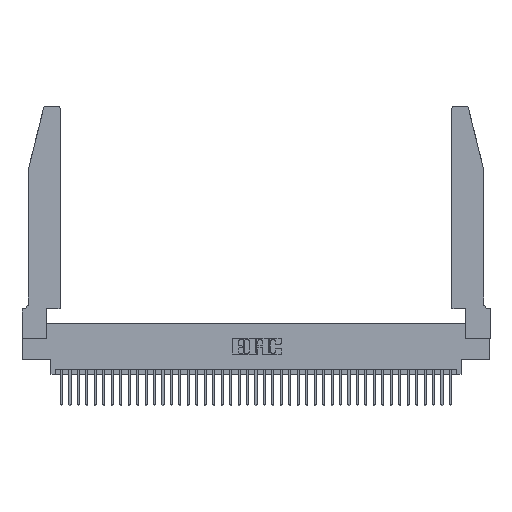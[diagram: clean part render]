
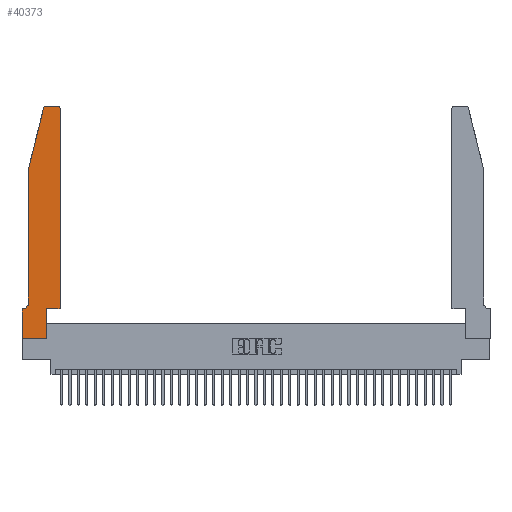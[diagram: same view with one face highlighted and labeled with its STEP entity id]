
A CAD part, top view. The second image highlights one B-rep face of the part: STEP entity #40373.
In plain terms, the highlighted planar face has unit normal (0, 0, 1).
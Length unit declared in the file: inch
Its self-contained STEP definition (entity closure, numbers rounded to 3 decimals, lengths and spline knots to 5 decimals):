
#163 = EDGE_CURVE ( 'NONE', #26604, #31561, #27139, .T. ) ;
#851 = DIRECTION ( 'NONE',  ( 0., -1., 0. ) ) ;
#1179 = AXIS2_PLACEMENT_3D ( 'NONE', #20336, #20608, #15203 ) ;
#2220 = CARTESIAN_POINT ( 'NONE',  ( 0.4505, 0.35, 0.37 ) ) ;
#2882 = VECTOR ( 'NONE', #851, 39.37008 ) ;
#3058 = ORIENTED_EDGE ( 'NONE', *, *, #35849, .T. ) ;
#3100 = ORIENTED_EDGE ( 'NONE', *, *, #12006, .T. ) ;
#3181 = VECTOR ( 'NONE', #8844, 39.37008 ) ;
#3531 = AXIS2_PLACEMENT_3D ( 'NONE', #12053, #40711, #15668 ) ;
#4727 = CIRCLE ( 'NONE', #17634, 0.03 ) ;
#4817 = LINE ( 'NONE', #2220, #30569 ) ;
#6264 = EDGE_CURVE ( 'NONE', #33062, #15789, #32249, .T. ) ;
#8247 = FACE_OUTER_BOUND ( 'NONE', #38529, .T. ) ;
#8464 = CARTESIAN_POINT ( 'NONE',  ( 0.2865, 0.35, 0.37 ) ) ;
#8844 = DIRECTION ( 'NONE',  ( -0.239, -0.971, 0. ) ) ;
#9478 = DIRECTION ( 'NONE',  ( 0., 0., 1. ) ) ;
#9781 = LINE ( 'NONE', #20766, #28170 ) ;
#10214 = CARTESIAN_POINT ( 'NONE',  ( 0.2865, 0., 0.37 ) ) ;
#10306 = ORIENTED_EDGE ( 'NONE', *, *, #33803, .T. ) ;
#11037 = EDGE_CURVE ( 'NONE', #12866, #26750, #38738, .T. ) ;
#11564 = LINE ( 'NONE', #15688, #3181 ) ;
#11738 = CARTESIAN_POINT ( 'NONE',  ( 0.284, 2.75, 0.37 ) ) ;
#12006 = EDGE_CURVE ( 'NONE', #15789, #32274, #9781, .T. ) ;
#12053 = CARTESIAN_POINT ( 'NONE',  ( 0.284, 2.72, 0.37 ) ) ;
#12736 = VECTOR ( 'NONE', #32404, 39.37008 ) ;
#12862 = CARTESIAN_POINT ( 'NONE',  ( 0.0755, 0.42, 0.37 ) ) ;
#12866 = VERTEX_POINT ( 'NONE', #11738 ) ;
#13192 = CARTESIAN_POINT ( 'NONE',  ( 0., 0., 0.37 ) ) ;
#13201 = DIRECTION ( 'NONE',  ( 1., 0., 0. ) ) ;
#13508 = EDGE_CURVE ( 'NONE', #40597, #20562, #4727, .T. ) ;
#13891 = VECTOR ( 'NONE', #28817, 39.37008 ) ;
#14452 = EDGE_CURVE ( 'NONE', #31561, #14847, #39031, .T. ) ;
#14701 = CARTESIAN_POINT ( 'NONE',  ( 0., 0., 0.37 ) ) ;
#14847 = VERTEX_POINT ( 'NONE', #26320 ) ;
#15076 = CARTESIAN_POINT ( 'NONE',  ( 0.0755, 0.35, 0.37 ) ) ;
#15203 = DIRECTION ( 'NONE',  ( -1., 0., 0. ) ) ;
#15668 = DIRECTION ( 'NONE',  ( 1., 0., 0. ) ) ;
#15688 = CARTESIAN_POINT ( 'NONE',  ( 0.0755, 2., 0.37 ) ) ;
#15789 = VERTEX_POINT ( 'NONE', #19706 ) ;
#15852 = EDGE_CURVE ( 'NONE', #20562, #12866, #21343, .T. ) ;
#16267 = CARTESIAN_POINT ( 'NONE',  ( 0.0055, 0.35, 0.37 ) ) ;
#16321 = VECTOR ( 'NONE', #18059, 39.37008 ) ;
#16983 = LINE ( 'NONE', #38303, #32938 ) ;
#17210 = CARTESIAN_POINT ( 'NONE',  ( 0.4505, 2.72, 0.37 ) ) ;
#17634 = AXIS2_PLACEMENT_3D ( 'NONE', #29583, #9478, #19070 ) ;
#18059 = DIRECTION ( 'NONE',  ( 0., 1., 0. ) ) ;
#18620 = EDGE_CURVE ( 'NONE', #32274, #40597, #4817, .T. ) ;
#19070 = DIRECTION ( 'NONE',  ( 1., 0., 0. ) ) ;
#19706 = CARTESIAN_POINT ( 'NONE',  ( 0.2865, 0.35, 0.37 ) ) ;
#19749 = CARTESIAN_POINT ( 'NONE',  ( 0.25487, 2.72718, 0.37 ) ) ;
#19924 = ORIENTED_EDGE ( 'NONE', *, *, #24065, .T. ) ;
#20336 = CARTESIAN_POINT ( 'NONE',  ( 0.0055, 0.42, 0.37 ) ) ;
#20340 = ORIENTED_EDGE ( 'NONE', *, *, #14452, .T. ) ;
#20562 = VERTEX_POINT ( 'NONE', #31272 ) ;
#20608 = DIRECTION ( 'NONE',  ( 0., 0., -1. ) ) ;
#20708 = ORIENTED_EDGE ( 'NONE', *, *, #11037, .T. ) ;
#20766 = CARTESIAN_POINT ( 'NONE',  ( 0.4505, 0.35, 0.37 ) ) ;
#21343 = LINE ( 'NONE', #28571, #13891 ) ;
#22467 = VECTOR ( 'NONE', #24518, 39.37008 ) ;
#23206 = DIRECTION ( 'NONE',  ( 0., 0., 1. ) ) ;
#23241 = DIRECTION ( 'NONE',  ( 0., 1., 0. ) ) ;
#23351 = ORIENTED_EDGE ( 'NONE', *, *, #6264, .T. ) ;
#24065 = EDGE_CURVE ( 'NONE', #14847, #32064, #39143, .T. ) ;
#24209 = ORIENTED_EDGE ( 'NONE', *, *, #15852, .T. ) ;
#24518 = DIRECTION ( 'NONE',  ( -1., 0., 0. ) ) ;
#25162 = EDGE_CURVE ( 'NONE', #32064, #33062, #28608, .T. ) ;
#26092 = CARTESIAN_POINT ( 'NONE',  ( 0., 0.35, 0.37 ) ) ;
#26320 = CARTESIAN_POINT ( 'NONE',  ( 0., 0.35, 0.37 ) ) ;
#26604 = VERTEX_POINT ( 'NONE', #12862 ) ;
#26750 = VERTEX_POINT ( 'NONE', #19749 ) ;
#27139 = CIRCLE ( 'NONE', #1179, 0.07 ) ;
#27492 = ORIENTED_EDGE ( 'NONE', *, *, #25162, .T. ) ;
#28170 = VECTOR ( 'NONE', #30614, 39.37008 ) ;
#28571 = CARTESIAN_POINT ( 'NONE',  ( 0.2605, 2.75, 0.37 ) ) ;
#28608 = LINE ( 'NONE', #13192, #12736 ) ;
#28817 = DIRECTION ( 'NONE',  ( -1., 0., 0. ) ) ;
#28919 = VERTEX_POINT ( 'NONE', #36208 ) ;
#29583 = CARTESIAN_POINT ( 'NONE',  ( 0.4205, 2.72, 0.37 ) ) ;
#30569 = VECTOR ( 'NONE', #23241, 39.37008 ) ;
#30614 = DIRECTION ( 'NONE',  ( 1., 0., 0. ) ) ;
#31272 = CARTESIAN_POINT ( 'NONE',  ( 0.4205, 2.75, 0.37 ) ) ;
#31301 = AXIS2_PLACEMENT_3D ( 'NONE', #26092, #23206, #13201 ) ;
#31561 = VERTEX_POINT ( 'NONE', #16267 ) ;
#31822 = CARTESIAN_POINT ( 'NONE',  ( 0.4505, 0.35, 0.37 ) ) ;
#32064 = VERTEX_POINT ( 'NONE', #14701 ) ;
#32249 = LINE ( 'NONE', #8464, #16321 ) ;
#32274 = VERTEX_POINT ( 'NONE', #31822 ) ;
#32404 = DIRECTION ( 'NONE',  ( 1., 0., 0. ) ) ;
#32434 = DIRECTION ( 'NONE',  ( 0., -1., 0. ) ) ;
#32938 = VECTOR ( 'NONE', #32434, 39.37008 ) ;
#33062 = VERTEX_POINT ( 'NONE', #10214 ) ;
#33803 = EDGE_CURVE ( 'NONE', #28919, #26604, #16983, .T. ) ;
#34806 = ORIENTED_EDGE ( 'NONE', *, *, #18620, .T. ) ;
#35849 = EDGE_CURVE ( 'NONE', #26750, #28919, #11564, .T. ) ;
#35903 = PLANE ( 'NONE',  #31301 ) ;
#36208 = CARTESIAN_POINT ( 'NONE',  ( 0.0755, 2., 0.37 ) ) ;
#37728 = ORIENTED_EDGE ( 'NONE', *, *, #163, .T. ) ;
#38303 = CARTESIAN_POINT ( 'NONE',  ( 0.0755, 2., 0.37 ) ) ;
#38529 = EDGE_LOOP ( 'NONE', ( #24209, #20708, #3058, #10306, #37728, #20340, #19924, #27492, #23351, #3100, #34806, #40014 ) ) ;
#38738 = CIRCLE ( 'NONE', #3531, 0.03 ) ;
#39031 = LINE ( 'NONE', #15076, #22467 ) ;
#39143 = LINE ( 'NONE', #41075, #2882 ) ;
#40014 = ORIENTED_EDGE ( 'NONE', *, *, #13508, .T. ) ;
#40373 = ADVANCED_FACE ( 'NONE', ( #8247 ), #35903, .T. ) ;
#40597 = VERTEX_POINT ( 'NONE', #17210 ) ;
#40711 = DIRECTION ( 'NONE',  ( 0., 0., 1. ) ) ;
#41075 = CARTESIAN_POINT ( 'NONE',  ( 0., 0., 0.37 ) ) ;
